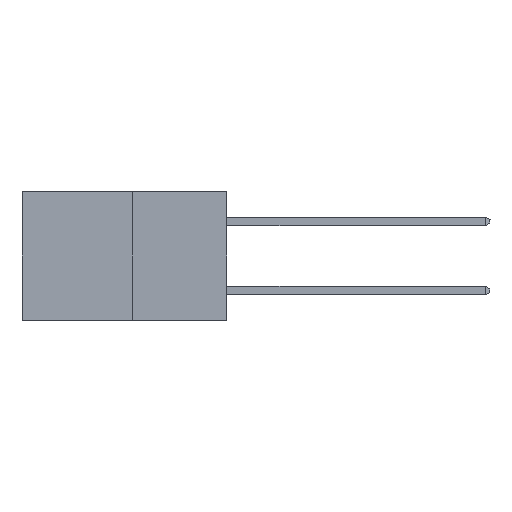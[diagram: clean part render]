
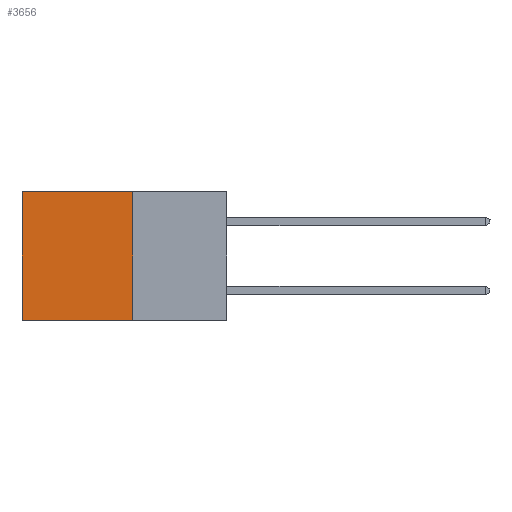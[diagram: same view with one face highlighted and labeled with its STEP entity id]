
A CAD part, left-side view. The second image highlights one B-rep face of the part: STEP entity #3656.
In plain terms, the highlighted planar face has unit normal (-1, 0, 0).
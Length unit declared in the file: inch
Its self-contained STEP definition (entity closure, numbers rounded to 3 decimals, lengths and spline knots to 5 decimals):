
#973 = VERTEX_POINT ( 'NONE', #9939 ) ;
#1069 = DIRECTION ( 'NONE',  ( 0., 1., 0. ) ) ;
#2142 = EDGE_LOOP ( 'NONE', ( #3125, #11627, #6634, #5883 ) ) ;
#2368 = VECTOR ( 'NONE', #4526, 39.37008 ) ;
#3017 = VERTEX_POINT ( 'NONE', #9741 ) ;
#3125 = ORIENTED_EDGE ( 'NONE', *, *, #7641, .T. ) ;
#3550 = DIRECTION ( 'NONE',  ( 1., 0., 0. ) ) ;
#3656 = ADVANCED_FACE ( 'NONE', ( #8892 ), #4348, .F. ) ;
#4329 = VECTOR ( 'NONE', #1069, 39.37008 ) ;
#4348 = PLANE ( 'NONE',  #13361 ) ;
#4526 = DIRECTION ( 'NONE',  ( 0., 1., 0. ) ) ;
#5489 = CARTESIAN_POINT ( 'NONE',  ( 0.277, 0.27, -0.37 ) ) ;
#5883 = ORIENTED_EDGE ( 'NONE', *, *, #10569, .T. ) ;
#6273 = VERTEX_POINT ( 'NONE', #7431 ) ;
#6417 = CARTESIAN_POINT ( 'NONE',  ( 0.277, 0.27, -0.37 ) ) ;
#6634 = ORIENTED_EDGE ( 'NONE', *, *, #11897, .F. ) ;
#6644 = LINE ( 'NONE', #6417, #4329 ) ;
#7114 = VERTEX_POINT ( 'NONE', #12485 ) ;
#7340 = CARTESIAN_POINT ( 'NONE',  ( 0.277, 0.27, -0.37 ) ) ;
#7431 = CARTESIAN_POINT ( 'NONE',  ( 0.277, 0.27, -0.37 ) ) ;
#7589 = LINE ( 'NONE', #7340, #7923 ) ;
#7641 = EDGE_CURVE ( 'NONE', #7114, #973, #11274, .T. ) ;
#7923 = VECTOR ( 'NONE', #9375, 39.37008 ) ;
#8255 = DIRECTION ( 'NONE',  ( 0., 0., -1. ) ) ;
#8259 = DIRECTION ( 'NONE',  ( 0., 0., -1. ) ) ;
#8892 = FACE_OUTER_BOUND ( 'NONE', #2142, .T. ) ;
#9375 = DIRECTION ( 'NONE',  ( 0., 0., -1. ) ) ;
#9741 = CARTESIAN_POINT ( 'NONE',  ( 0.277, 0.27, 0. ) ) ;
#9939 = CARTESIAN_POINT ( 'NONE',  ( 0.277, 0.59, -0.37 ) ) ;
#10569 = EDGE_CURVE ( 'NONE', #3017, #7114, #11210, .T. ) ;
#11210 = LINE ( 'NONE', #11508, #2368 ) ;
#11274 = LINE ( 'NONE', #13116, #13198 ) ;
#11508 = CARTESIAN_POINT ( 'NONE',  ( 0.277, 0.27, 0. ) ) ;
#11627 = ORIENTED_EDGE ( 'NONE', *, *, #11996, .F. ) ;
#11897 = EDGE_CURVE ( 'NONE', #3017, #6273, #7589, .T. ) ;
#11996 = EDGE_CURVE ( 'NONE', #6273, #973, #6644, .T. ) ;
#12485 = CARTESIAN_POINT ( 'NONE',  ( 0.277, 0.59, 0. ) ) ;
#13116 = CARTESIAN_POINT ( 'NONE',  ( 0.277, 0.59, -0.37 ) ) ;
#13198 = VECTOR ( 'NONE', #8255, 39.37008 ) ;
#13361 = AXIS2_PLACEMENT_3D ( 'NONE', #5489, #3550, #8259 ) ;
